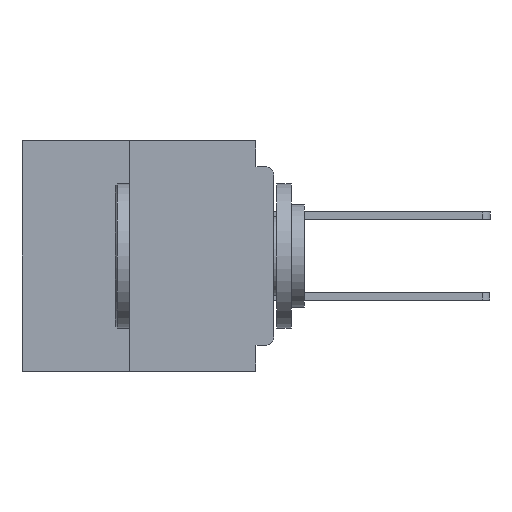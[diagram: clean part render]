
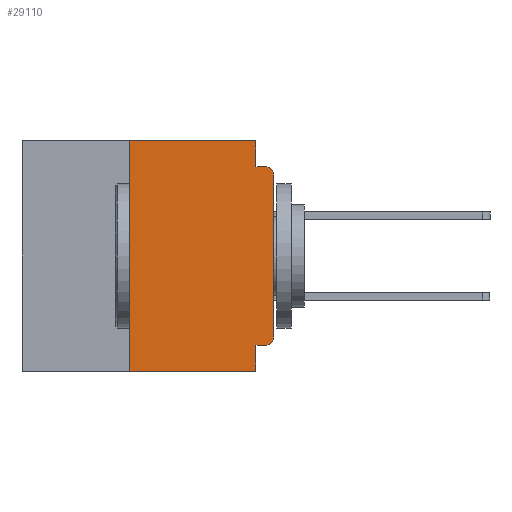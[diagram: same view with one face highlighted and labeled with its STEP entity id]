
A CAD part, left-side view. The second image highlights one B-rep face of the part: STEP entity #29110.
In plain terms, the highlighted planar face has unit normal (-1, 0, 0).
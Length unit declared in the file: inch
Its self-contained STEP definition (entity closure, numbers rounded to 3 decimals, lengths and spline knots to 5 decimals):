
#916 = ORIENTED_EDGE ( 'NONE', *, *, #8921, .F. ) ;
#1049 = VERTEX_POINT ( 'NONE', #13894 ) ;
#1307 = CARTESIAN_POINT ( 'NONE',  ( 0., 0.437, 0. ) ) ;
#1460 = ORIENTED_EDGE ( 'NONE', *, *, #34186, .F. ) ;
#1880 = AXIS2_PLACEMENT_3D ( 'NONE', #1307, #33167, #14392 ) ;
#2335 = AXIS2_PLACEMENT_3D ( 'NONE', #25772, #6738, #28928 ) ;
#3500 = ORIENTED_EDGE ( 'NONE', *, *, #40848, .F. ) ;
#3559 = VECTOR ( 'NONE', #12756, 39.37008 ) ;
#4290 = CARTESIAN_POINT ( 'NONE',  ( 0., 0.015, -0.355 ) ) ;
#4349 = EDGE_CURVE ( 'NONE', #1049, #37560, #23763, .T. ) ;
#5133 = VECTOR ( 'NONE', #8107, 39.37008 ) ;
#5279 = VECTOR ( 'NONE', #13669, 39.37008 ) ;
#5494 = EDGE_CURVE ( 'NONE', #22374, #38123, #6133, .T. ) ;
#6133 = LINE ( 'NONE', #7673, #5133 ) ;
#6738 = DIRECTION ( 'NONE',  ( -1., 0., 0. ) ) ;
#6856 = DIRECTION ( 'NONE',  ( 0., 0., -1. ) ) ;
#7065 = ORIENTED_EDGE ( 'NONE', *, *, #15486, .F. ) ;
#7569 = ORIENTED_EDGE ( 'NONE', *, *, #4349, .F. ) ;
#7673 = CARTESIAN_POINT ( 'NONE',  ( 0., 0.437, 0. ) ) ;
#7799 = VECTOR ( 'NONE', #17770, 39.37008 ) ;
#8107 = DIRECTION ( 'NONE',  ( 0., -1., 0. ) ) ;
#8921 = EDGE_CURVE ( 'NONE', #38123, #1049, #19839, .T. ) ;
#9252 = LINE ( 'NONE', #21271, #17760 ) ;
#9737 = CARTESIAN_POINT ( 'NONE',  ( 0., 0.015, -0.06 ) ) ;
#10397 = CARTESIAN_POINT ( 'NONE',  ( 0., 0.25, -0.4 ) ) ;
#11168 = CARTESIAN_POINT ( 'NONE',  ( 0., 0.031, -0.4 ) ) ;
#11568 = AXIS2_PLACEMENT_3D ( 'NONE', #9737, #31792, #12982 ) ;
#12584 = CARTESIAN_POINT ( 'NONE',  ( 0., 0., -0.06 ) ) ;
#12756 = DIRECTION ( 'NONE',  ( 0., 1., 0. ) ) ;
#12982 = DIRECTION ( 'NONE',  ( 0., 0., -1. ) ) ;
#13669 = DIRECTION ( 'NONE',  ( 0., 0., 1. ) ) ;
#13894 = CARTESIAN_POINT ( 'NONE',  ( 0., 0.031, -0.045 ) ) ;
#13922 = LINE ( 'NONE', #10397, #5279 ) ;
#14017 = CARTESIAN_POINT ( 'NONE',  ( 0., 0.25, -0.4 ) ) ;
#14392 = DIRECTION ( 'NONE',  ( 0., 0., -1. ) ) ;
#14423 = DIRECTION ( 'NONE',  ( 0., 0., -1. ) ) ;
#15229 = VERTEX_POINT ( 'NONE', #25095 ) ;
#15486 = EDGE_CURVE ( 'NONE', #22840, #22374, #13922, .T. ) ;
#16914 = LINE ( 'NONE', #11168, #31600 ) ;
#17042 = CARTESIAN_POINT ( 'NONE',  ( 0., 0.031, -0.4 ) ) ;
#17760 = VECTOR ( 'NONE', #21135, 39.37008 ) ;
#17770 = DIRECTION ( 'NONE',  ( 0., -1., 0. ) ) ;
#17960 = ORIENTED_EDGE ( 'NONE', *, *, #34589, .T. ) ;
#18029 = EDGE_LOOP ( 'NONE', ( #24002, #38133, #7569, #916, #31333, #7065, #34279, #1460, #3500, #17960 ) ) ;
#18047 = CARTESIAN_POINT ( 'NONE',  ( 0., 0.25, 0. ) ) ;
#18170 = CARTESIAN_POINT ( 'NONE',  ( 0., 0., -0.045 ) ) ;
#18840 = CIRCLE ( 'NONE', #2335, 0.015 ) ;
#18845 = VERTEX_POINT ( 'NONE', #12584 ) ;
#18878 = CARTESIAN_POINT ( 'NONE',  ( 0., 0.015, -0.045 ) ) ;
#18910 = CARTESIAN_POINT ( 'NONE',  ( 0., 0.437, -0.4 ) ) ;
#19482 = EDGE_CURVE ( 'NONE', #22840, #34054, #38109, .T. ) ;
#19839 = LINE ( 'NONE', #29054, #27208 ) ;
#21135 = DIRECTION ( 'NONE',  ( 0., 0., 1. ) ) ;
#21271 = CARTESIAN_POINT ( 'NONE',  ( 0., 0., 0. ) ) ;
#22070 = DIRECTION ( 'NONE',  ( 0., -1., 0. ) ) ;
#22374 = VERTEX_POINT ( 'NONE', #18047 ) ;
#22840 = VERTEX_POINT ( 'NONE', #14017 ) ;
#23201 = FACE_OUTER_BOUND ( 'NONE', #18029, .T. ) ;
#23273 = EDGE_CURVE ( 'NONE', #18845, #37560, #24357, .T. ) ;
#23763 = LINE ( 'NONE', #18170, #7799 ) ;
#24002 = ORIENTED_EDGE ( 'NONE', *, *, #25349, .T. ) ;
#24357 = CIRCLE ( 'NONE', #11568, 0.015 ) ;
#25015 = CARTESIAN_POINT ( 'NONE',  ( 0., 0.031, 0. ) ) ;
#25095 = CARTESIAN_POINT ( 'NONE',  ( 0., 0.031, -0.355 ) ) ;
#25349 = EDGE_CURVE ( 'NONE', #35180, #18845, #9252, .T. ) ;
#25442 = CARTESIAN_POINT ( 'NONE',  ( 0., 0., -0.34 ) ) ;
#25772 = CARTESIAN_POINT ( 'NONE',  ( 0., 0.015, -0.34 ) ) ;
#27208 = VECTOR ( 'NONE', #6856, 39.37008 ) ;
#28928 = DIRECTION ( 'NONE',  ( 0., 0., -1. ) ) ;
#29054 = CARTESIAN_POINT ( 'NONE',  ( 0., 0.031, 0. ) ) ;
#29110 = ADVANCED_FACE ( 'NONE', ( #23201 ), #30042, .F. ) ;
#30042 = PLANE ( 'NONE',  #1880 ) ;
#31333 = ORIENTED_EDGE ( 'NONE', *, *, #5494, .F. ) ;
#31587 = CARTESIAN_POINT ( 'NONE',  ( 0., 0., -0.355 ) ) ;
#31600 = VECTOR ( 'NONE', #14423, 39.37008 ) ;
#31792 = DIRECTION ( 'NONE',  ( -1., 0., 0. ) ) ;
#33167 = DIRECTION ( 'NONE',  ( 1., 0., 0. ) ) ;
#34054 = VERTEX_POINT ( 'NONE', #17042 ) ;
#34186 = EDGE_CURVE ( 'NONE', #15229, #34054, #16914, .T. ) ;
#34279 = ORIENTED_EDGE ( 'NONE', *, *, #19482, .T. ) ;
#34589 = EDGE_CURVE ( 'NONE', #37355, #35180, #18840, .T. ) ;
#35180 = VERTEX_POINT ( 'NONE', #25442 ) ;
#35307 = LINE ( 'NONE', #31587, #3559 ) ;
#37139 = VECTOR ( 'NONE', #22070, 39.37008 ) ;
#37355 = VERTEX_POINT ( 'NONE', #4290 ) ;
#37560 = VERTEX_POINT ( 'NONE', #18878 ) ;
#38109 = LINE ( 'NONE', #18910, #37139 ) ;
#38123 = VERTEX_POINT ( 'NONE', #25015 ) ;
#38133 = ORIENTED_EDGE ( 'NONE', *, *, #23273, .T. ) ;
#40848 = EDGE_CURVE ( 'NONE', #37355, #15229, #35307, .T. ) ;
